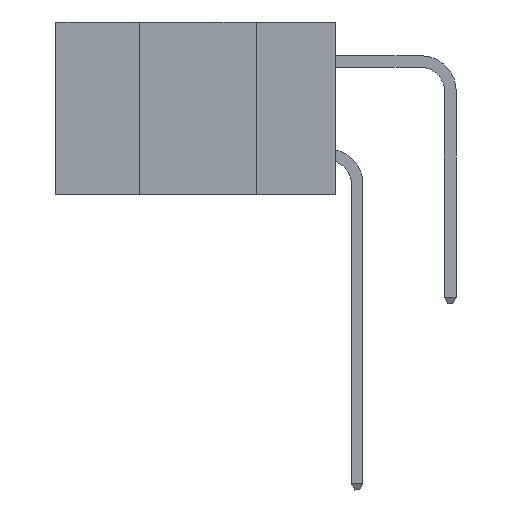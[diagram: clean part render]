
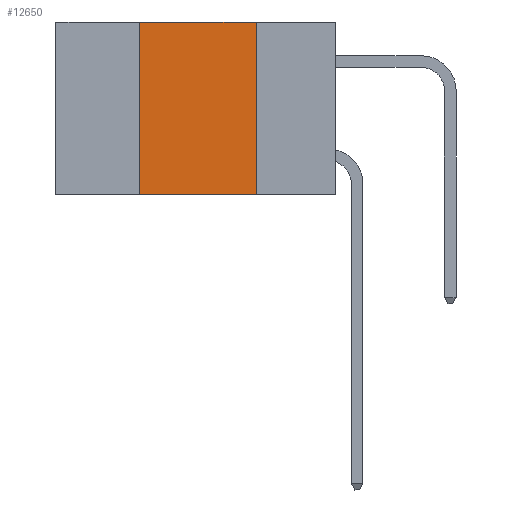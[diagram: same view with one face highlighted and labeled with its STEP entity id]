
A CAD part, left-side view. The second image highlights one B-rep face of the part: STEP entity #12650.
In plain terms, the highlighted planar face has unit normal (-1, 0, 0).
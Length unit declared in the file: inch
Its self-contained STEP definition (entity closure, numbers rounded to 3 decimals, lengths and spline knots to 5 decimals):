
#548 = VECTOR ( 'NONE', #7128, 39.37008 ) ;
#624 = EDGE_CURVE ( 'NONE', #21755, #2714, #15550, .T. ) ;
#2426 = LINE ( 'NONE', #16590, #10671 ) ;
#2714 = VERTEX_POINT ( 'NONE', #16250 ) ;
#2919 = PLANE ( 'NONE',  #24293 ) ;
#3151 = DIRECTION ( 'NONE',  ( 0., 0., -1. ) ) ;
#3426 = VERTEX_POINT ( 'NONE', #13006 ) ;
#3462 = DIRECTION ( 'NONE',  ( 0., 0., 1. ) ) ;
#3523 = VECTOR ( 'NONE', #11195, 39.37008 ) ;
#6830 = DIRECTION ( 'NONE',  ( 1., 0., 0. ) ) ;
#6971 = DIRECTION ( 'NONE',  ( 0., 0., -1. ) ) ;
#7128 = DIRECTION ( 'NONE',  ( 0., -1., 0. ) ) ;
#7748 = EDGE_CURVE ( 'NONE', #3426, #21755, #23654, .T. ) ;
#9441 = CARTESIAN_POINT ( 'NONE',  ( 0., 0.17, -0.37 ) ) ;
#10671 = VECTOR ( 'NONE', #6971, 39.37008 ) ;
#11195 = DIRECTION ( 'NONE',  ( 0., -1., 0. ) ) ;
#12650 = ADVANCED_FACE ( 'NONE', ( #18298 ), #2919, .F. ) ;
#13006 = CARTESIAN_POINT ( 'NONE',  ( 0., 0.42, -0.37 ) ) ;
#14051 = ORIENTED_EDGE ( 'NONE', *, *, #14690, .T. ) ;
#14618 = CARTESIAN_POINT ( 'NONE',  ( 0., 0.42, 0. ) ) ;
#14690 = EDGE_CURVE ( 'NONE', #3426, #16335, #19072, .T. ) ;
#15012 = ORIENTED_EDGE ( 'NONE', *, *, #7748, .F. ) ;
#15550 = LINE ( 'NONE', #18132, #548 ) ;
#16250 = CARTESIAN_POINT ( 'NONE',  ( 0., 0.17, 0. ) ) ;
#16335 = VERTEX_POINT ( 'NONE', #9441 ) ;
#16590 = CARTESIAN_POINT ( 'NONE',  ( 0., 0.17, 0. ) ) ;
#16941 = ORIENTED_EDGE ( 'NONE', *, *, #17376, .F. ) ;
#17376 = EDGE_CURVE ( 'NONE', #2714, #16335, #2426, .T. ) ;
#17471 = EDGE_LOOP ( 'NONE', ( #16941, #17639, #15012, #14051 ) ) ;
#17639 = ORIENTED_EDGE ( 'NONE', *, *, #624, .F. ) ;
#17993 = CARTESIAN_POINT ( 'NONE',  ( 0., 0.6, 0. ) ) ;
#18132 = CARTESIAN_POINT ( 'NONE',  ( 0., 0.6, 0. ) ) ;
#18298 = FACE_OUTER_BOUND ( 'NONE', #17471, .T. ) ;
#19072 = LINE ( 'NONE', #23948, #3523 ) ;
#20209 = CARTESIAN_POINT ( 'NONE',  ( 0., 0.42, 0. ) ) ;
#21320 = VECTOR ( 'NONE', #3462, 39.37008 ) ;
#21755 = VERTEX_POINT ( 'NONE', #20209 ) ;
#23654 = LINE ( 'NONE', #14618, #21320 ) ;
#23948 = CARTESIAN_POINT ( 'NONE',  ( 0., 0.6, -0.37 ) ) ;
#24293 = AXIS2_PLACEMENT_3D ( 'NONE', #17993, #6830, #3151 ) ;
